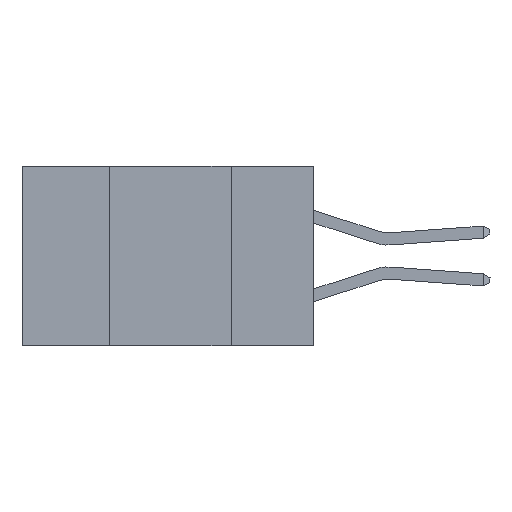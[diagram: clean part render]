
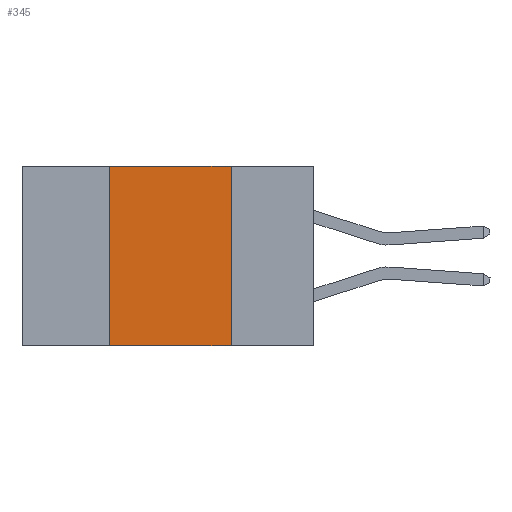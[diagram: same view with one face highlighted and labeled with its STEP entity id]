
A CAD part, left-side view. The second image highlights one B-rep face of the part: STEP entity #345.
In plain terms, the highlighted planar face has unit normal (-1, 0, 0).
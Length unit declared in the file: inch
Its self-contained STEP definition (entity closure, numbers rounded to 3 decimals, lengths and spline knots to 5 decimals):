
#345 = ADVANCED_FACE ( 'NONE', ( #13804 ), #9259, .F. ) ;
#868 = DIRECTION ( 'NONE',  ( 0., 0., -1. ) ) ;
#911 = ORIENTED_EDGE ( 'NONE', *, *, #17294, .F. ) ;
#1487 = VECTOR ( 'NONE', #3002, 39.37008 ) ;
#1747 = CARTESIAN_POINT ( 'NONE',  ( 0., 0.6, -0.37 ) ) ;
#2869 = VECTOR ( 'NONE', #14830, 39.37008 ) ;
#3002 = DIRECTION ( 'NONE',  ( 0., 0., 1. ) ) ;
#3611 = VERTEX_POINT ( 'NONE', #6487 ) ;
#4199 = EDGE_CURVE ( 'NONE', #3611, #9427, #10238, .T. ) ;
#5199 = EDGE_CURVE ( 'NONE', #12066, #9427, #5321, .T. ) ;
#5321 = LINE ( 'NONE', #9239, #2869 ) ;
#6004 = EDGE_CURVE ( 'NONE', #7117, #12066, #8238, .T. ) ;
#6487 = CARTESIAN_POINT ( 'NONE',  ( 0., 0.42, -0.37 ) ) ;
#6493 = CARTESIAN_POINT ( 'NONE',  ( 0., 0.6, 0. ) ) ;
#7117 = VERTEX_POINT ( 'NONE', #8212 ) ;
#8212 = CARTESIAN_POINT ( 'NONE',  ( 0., 0.42, 0. ) ) ;
#8238 = LINE ( 'NONE', #12104, #17693 ) ;
#8540 = DIRECTION ( 'NONE',  ( 0., -1., 0. ) ) ;
#8610 = CARTESIAN_POINT ( 'NONE',  ( 0., 0.42, 0. ) ) ;
#9239 = CARTESIAN_POINT ( 'NONE',  ( 0., 0.17, 0. ) ) ;
#9259 = PLANE ( 'NONE',  #10649 ) ;
#9427 = VERTEX_POINT ( 'NONE', #14814 ) ;
#10238 = LINE ( 'NONE', #1747, #13092 ) ;
#10649 = AXIS2_PLACEMENT_3D ( 'NONE', #6493, #16291, #868 ) ;
#11972 = DIRECTION ( 'NONE',  ( 0., -1., 0. ) ) ;
#12066 = VERTEX_POINT ( 'NONE', #15323 ) ;
#12104 = CARTESIAN_POINT ( 'NONE',  ( 0., 0.6, 0. ) ) ;
#12544 = ORIENTED_EDGE ( 'NONE', *, *, #5199, .F. ) ;
#13092 = VECTOR ( 'NONE', #8540, 39.37008 ) ;
#13348 = ORIENTED_EDGE ( 'NONE', *, *, #6004, .F. ) ;
#13804 = FACE_OUTER_BOUND ( 'NONE', #15835, .T. ) ;
#14814 = CARTESIAN_POINT ( 'NONE',  ( 0., 0.17, -0.37 ) ) ;
#14830 = DIRECTION ( 'NONE',  ( 0., 0., -1. ) ) ;
#15323 = CARTESIAN_POINT ( 'NONE',  ( 0., 0.17, 0. ) ) ;
#15351 = LINE ( 'NONE', #8610, #1487 ) ;
#15835 = EDGE_LOOP ( 'NONE', ( #12544, #13348, #911, #16952 ) ) ;
#16291 = DIRECTION ( 'NONE',  ( 1., 0., 0. ) ) ;
#16952 = ORIENTED_EDGE ( 'NONE', *, *, #4199, .T. ) ;
#17294 = EDGE_CURVE ( 'NONE', #3611, #7117, #15351, .T. ) ;
#17693 = VECTOR ( 'NONE', #11972, 39.37008 ) ;
